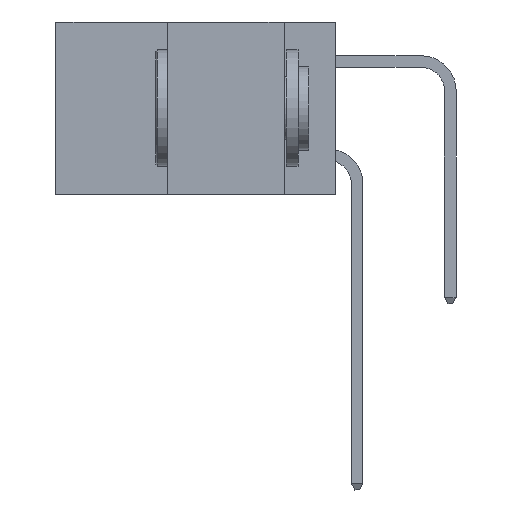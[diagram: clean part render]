
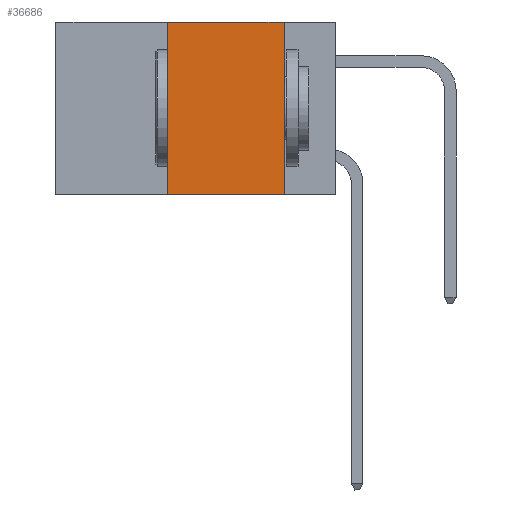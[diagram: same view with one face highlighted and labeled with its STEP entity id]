
A CAD part, left-side view. The second image highlights one B-rep face of the part: STEP entity #36686.
In plain terms, the highlighted planar face has unit normal (-1, 0, 0).
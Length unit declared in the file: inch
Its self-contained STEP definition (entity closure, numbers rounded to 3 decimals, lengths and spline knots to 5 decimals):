
#215 = CARTESIAN_POINT ( 'NONE',  ( 0., 0.36, 0. ) ) ;
#497 = CARTESIAN_POINT ( 'NONE',  ( 0., 0.6, 0. ) ) ;
#2287 = LINE ( 'NONE', #29803, #32058 ) ;
#3165 = LINE ( 'NONE', #28133, #33894 ) ;
#3252 = FACE_OUTER_BOUND ( 'NONE', #21682, .T. ) ;
#4303 = EDGE_CURVE ( 'NONE', #25769, #5245, #35549, .T. ) ;
#4328 = CARTESIAN_POINT ( 'NONE',  ( 0., 0.11, -0.37 ) ) ;
#4508 = ORIENTED_EDGE ( 'NONE', *, *, #26495, .F. ) ;
#5213 = LINE ( 'NONE', #497, #35945 ) ;
#5245 = VERTEX_POINT ( 'NONE', #4328 ) ;
#6434 = ORIENTED_EDGE ( 'NONE', *, *, #4303, .T. ) ;
#7235 = CARTESIAN_POINT ( 'NONE',  ( 0., 0.36, -0.37 ) ) ;
#7431 = DIRECTION ( 'NONE',  ( 0., 0., -1. ) ) ;
#8890 = DIRECTION ( 'NONE',  ( 0., -1., 0. ) ) ;
#9138 = DIRECTION ( 'NONE',  ( 0., 0., 1. ) ) ;
#13404 = ORIENTED_EDGE ( 'NONE', *, *, #24633, .F. ) ;
#15584 = DIRECTION ( 'NONE',  ( 0., -1., 0. ) ) ;
#16925 = CARTESIAN_POINT ( 'NONE',  ( 0., 0.6, 0. ) ) ;
#19879 = DIRECTION ( 'NONE',  ( 0., 0., -1. ) ) ;
#21682 = EDGE_LOOP ( 'NONE', ( #4508, #13404, #29126, #6434 ) ) ;
#24633 = EDGE_CURVE ( 'NONE', #32929, #27769, #5213, .T. ) ;
#25769 = VERTEX_POINT ( 'NONE', #7235 ) ;
#26495 = EDGE_CURVE ( 'NONE', #27769, #5245, #3165, .T. ) ;
#26626 = CARTESIAN_POINT ( 'NONE',  ( 0., 0.6, -0.37 ) ) ;
#27442 = AXIS2_PLACEMENT_3D ( 'NONE', #16925, #37699, #19879 ) ;
#27571 = VECTOR ( 'NONE', #8890, 39.37008 ) ;
#27769 = VERTEX_POINT ( 'NONE', #28354 ) ;
#28133 = CARTESIAN_POINT ( 'NONE',  ( 0., 0.11, 0. ) ) ;
#28354 = CARTESIAN_POINT ( 'NONE',  ( 0., 0.11, 0. ) ) ;
#29126 = ORIENTED_EDGE ( 'NONE', *, *, #34980, .F. ) ;
#29803 = CARTESIAN_POINT ( 'NONE',  ( 0., 0.36, 0. ) ) ;
#31644 = PLANE ( 'NONE',  #27442 ) ;
#32058 = VECTOR ( 'NONE', #9138, 39.37008 ) ;
#32929 = VERTEX_POINT ( 'NONE', #215 ) ;
#33894 = VECTOR ( 'NONE', #7431, 39.37008 ) ;
#34980 = EDGE_CURVE ( 'NONE', #25769, #32929, #2287, .T. ) ;
#35549 = LINE ( 'NONE', #26626, #27571 ) ;
#35945 = VECTOR ( 'NONE', #15584, 39.37008 ) ;
#36686 = ADVANCED_FACE ( 'NONE', ( #3252 ), #31644, .F. ) ;
#37699 = DIRECTION ( 'NONE',  ( 1., 0., 0. ) ) ;
